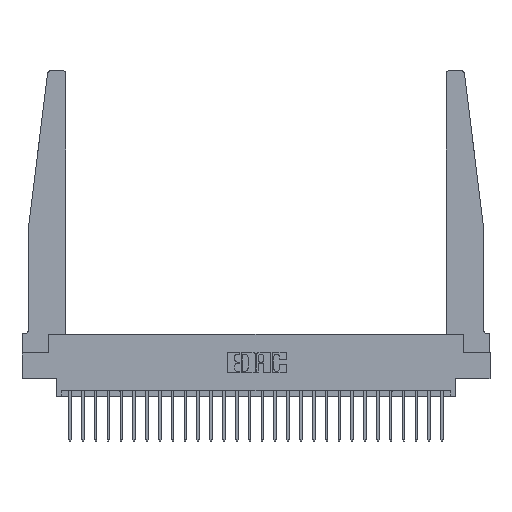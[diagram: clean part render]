
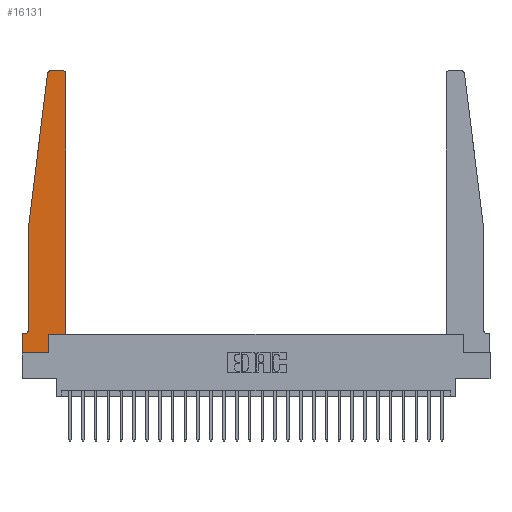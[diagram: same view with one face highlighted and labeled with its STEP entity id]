
A CAD part, top view. The second image highlights one B-rep face of the part: STEP entity #16131.
In plain terms, the highlighted planar face has unit normal (0, 0, 1).
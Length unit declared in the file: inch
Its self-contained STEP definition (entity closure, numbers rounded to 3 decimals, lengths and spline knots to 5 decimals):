
#276 = VECTOR ( 'NONE', #16497, 39.37008 ) ;
#402 = EDGE_CURVE ( 'NONE', #14051, #10019, #10716, .T. ) ;
#574 = ORIENTED_EDGE ( 'NONE', *, *, #2592, .T. ) ;
#743 = LINE ( 'NONE', #22726, #1393 ) ;
#865 = LINE ( 'NONE', #4766, #21819 ) ;
#1152 = CARTESIAN_POINT ( 'NONE',  ( 0.395, 2.75, 0.37 ) ) ;
#1393 = VECTOR ( 'NONE', #10576, 39.37008 ) ;
#1911 = EDGE_CURVE ( 'NONE', #15231, #13709, #19567, .T. ) ;
#2016 = AXIS2_PLACEMENT_3D ( 'NONE', #4565, #18829, #6612 ) ;
#2082 = VECTOR ( 'NONE', #21500, 39.37008 ) ;
#2258 = CARTESIAN_POINT ( 'NONE',  ( 0., 0., 0.37 ) ) ;
#2498 = ORIENTED_EDGE ( 'NONE', *, *, #7749, .T. ) ;
#2572 = CARTESIAN_POINT ( 'NONE',  ( 0., 0., 0.37 ) ) ;
#2592 = EDGE_CURVE ( 'NONE', #13709, #11650, #3611, .T. ) ;
#3297 = FACE_OUTER_BOUND ( 'NONE', #6999, .T. ) ;
#3611 = LINE ( 'NONE', #21758, #14441 ) ;
#3746 = ORIENTED_EDGE ( 'NONE', *, *, #12620, .T. ) ;
#4225 = CARTESIAN_POINT ( 'NONE',  ( 0., 0.1875, 0.37 ) ) ;
#4300 = VERTEX_POINT ( 'NONE', #16237 ) ;
#4429 = VECTOR ( 'NONE', #10445, 39.37008 ) ;
#4565 = CARTESIAN_POINT ( 'NONE',  ( 0.27653, 2.72, 0.37 ) ) ;
#4584 = DIRECTION ( 'NONE',  ( 0., -1., 0. ) ) ;
#4766 = CARTESIAN_POINT ( 'NONE',  ( 0.425, 0.18, 0.37 ) ) ;
#5009 = CARTESIAN_POINT ( 'NONE',  ( 0.015, 0.2375, 0.37 ) ) ;
#5012 = ORIENTED_EDGE ( 'NONE', *, *, #13566, .T. ) ;
#5018 = LINE ( 'NONE', #2258, #276 ) ;
#5101 = LINE ( 'NONE', #6433, #17252 ) ;
#5289 = AXIS2_PLACEMENT_3D ( 'NONE', #19246, #7040, #21251 ) ;
#5971 = ORIENTED_EDGE ( 'NONE', *, *, #9443, .T. ) ;
#6433 = CARTESIAN_POINT ( 'NONE',  ( 0.065, 1.25, 0.37 ) ) ;
#6599 = ORIENTED_EDGE ( 'NONE', *, *, #21748, .T. ) ;
#6612 = DIRECTION ( 'NONE',  ( 1., 0., 0. ) ) ;
#6999 = EDGE_LOOP ( 'NONE', ( #574, #5971, #6599, #12017, #22783, #2498, #13295, #3746, #9151, #19959, #5012, #15879 ) ) ;
#7040 = DIRECTION ( 'NONE',  ( 0., 0., 1. ) ) ;
#7749 = EDGE_CURVE ( 'NONE', #10019, #13974, #743, .T. ) ;
#7973 = CARTESIAN_POINT ( 'NONE',  ( 0., 0.1875, 0.37 ) ) ;
#8414 = CARTESIAN_POINT ( 'NONE',  ( 0.065, 1.25, 0.37 ) ) ;
#8613 = VERTEX_POINT ( 'NONE', #17256 ) ;
#8951 = EDGE_CURVE ( 'NONE', #20756, #14051, #5101, .T. ) ;
#9151 = ORIENTED_EDGE ( 'NONE', *, *, #14937, .T. ) ;
#9443 = EDGE_CURVE ( 'NONE', #11650, #11386, #11553, .T. ) ;
#9492 = VECTOR ( 'NONE', #4584, 39.37008 ) ;
#9989 = DIRECTION ( 'NONE',  ( 1., 0., 0. ) ) ;
#10019 = VERTEX_POINT ( 'NONE', #24514 ) ;
#10174 = CARTESIAN_POINT ( 'NONE',  ( 0.24675, 2.72367, 0.37 ) ) ;
#10445 = DIRECTION ( 'NONE',  ( -0.122, -0.992, 0. ) ) ;
#10576 = DIRECTION ( 'NONE',  ( -1., 0., 0. ) ) ;
#10716 = CIRCLE ( 'NONE', #11407, 0.05 ) ;
#11386 = VERTEX_POINT ( 'NONE', #10174 ) ;
#11407 = AXIS2_PLACEMENT_3D ( 'NONE', #5009, #18668, #23817 ) ;
#11553 = CIRCLE ( 'NONE', #2016, 0.03 ) ;
#11650 = VERTEX_POINT ( 'NONE', #21070 ) ;
#11752 = CARTESIAN_POINT ( 'NONE',  ( 0.065, 1.25, 0.37 ) ) ;
#11955 = PLANE ( 'NONE',  #14681 ) ;
#12017 = ORIENTED_EDGE ( 'NONE', *, *, #8951, .T. ) ;
#12620 = EDGE_CURVE ( 'NONE', #4300, #22200, #5018, .T. ) ;
#13295 = ORIENTED_EDGE ( 'NONE', *, *, #24982, .T. ) ;
#13436 = CARTESIAN_POINT ( 'NONE',  ( 0.2605, 0.18, 0.37 ) ) ;
#13566 = EDGE_CURVE ( 'NONE', #8613, #15231, #865, .T. ) ;
#13709 = VERTEX_POINT ( 'NONE', #1152 ) ;
#13938 = LINE ( 'NONE', #18996, #24018 ) ;
#13974 = VERTEX_POINT ( 'NONE', #4225 ) ;
#14051 = VERTEX_POINT ( 'NONE', #18653 ) ;
#14441 = VECTOR ( 'NONE', #23835, 39.37008 ) ;
#14681 = AXIS2_PLACEMENT_3D ( 'NONE', #7973, #22161, #9989 ) ;
#14937 = EDGE_CURVE ( 'NONE', #22200, #22851, #23606, .T. ) ;
#15231 = VERTEX_POINT ( 'NONE', #16384 ) ;
#15879 = ORIENTED_EDGE ( 'NONE', *, *, #1911, .T. ) ;
#15903 = CARTESIAN_POINT ( 'NONE',  ( 0.2605, 0., 0.37 ) ) ;
#16131 = ADVANCED_FACE ( 'NONE', ( #3297 ), #11955, .T. ) ;
#16237 = CARTESIAN_POINT ( 'NONE',  ( 0., 0., 0.37 ) ) ;
#16384 = CARTESIAN_POINT ( 'NONE',  ( 0.425, 2.72, 0.37 ) ) ;
#16497 = DIRECTION ( 'NONE',  ( 1., 0., 0. ) ) ;
#17252 = VECTOR ( 'NONE', #22672, 39.37008 ) ;
#17256 = CARTESIAN_POINT ( 'NONE',  ( 0.425, 0.18, 0.37 ) ) ;
#18190 = CARTESIAN_POINT ( 'NONE',  ( 0.2605, 0.18, 0.37 ) ) ;
#18653 = CARTESIAN_POINT ( 'NONE',  ( 0.065, 0.2375, 0.37 ) ) ;
#18668 = DIRECTION ( 'NONE',  ( 0., 0., -1. ) ) ;
#18829 = DIRECTION ( 'NONE',  ( 0., 0., 1. ) ) ;
#18996 = CARTESIAN_POINT ( 'NONE',  ( 0.425, 0.18, 0.37 ) ) ;
#19033 = DIRECTION ( 'NONE',  ( 0., 1., 0. ) ) ;
#19082 = DIRECTION ( 'NONE',  ( 1., 0., 0. ) ) ;
#19246 = CARTESIAN_POINT ( 'NONE',  ( 0.395, 2.72, 0.37 ) ) ;
#19401 = LINE ( 'NONE', #8414, #4429 ) ;
#19567 = CIRCLE ( 'NONE', #5289, 0.03 ) ;
#19959 = ORIENTED_EDGE ( 'NONE', *, *, #25769, .T. ) ;
#20756 = VERTEX_POINT ( 'NONE', #11752 ) ;
#21070 = CARTESIAN_POINT ( 'NONE',  ( 0.27653, 2.75, 0.37 ) ) ;
#21251 = DIRECTION ( 'NONE',  ( 1., 0., 0. ) ) ;
#21500 = DIRECTION ( 'NONE',  ( 0., 1., 0. ) ) ;
#21748 = EDGE_CURVE ( 'NONE', #11386, #20756, #19401, .T. ) ;
#21758 = CARTESIAN_POINT ( 'NONE',  ( 0.25, 2.75, 0.37 ) ) ;
#21819 = VECTOR ( 'NONE', #19033, 39.37008 ) ;
#22161 = DIRECTION ( 'NONE',  ( 0., 0., 1. ) ) ;
#22200 = VERTEX_POINT ( 'NONE', #15903 ) ;
#22672 = DIRECTION ( 'NONE',  ( 0., -1., 0. ) ) ;
#22726 = CARTESIAN_POINT ( 'NONE',  ( 0.065, 0.1875, 0.37 ) ) ;
#22783 = ORIENTED_EDGE ( 'NONE', *, *, #402, .T. ) ;
#22851 = VERTEX_POINT ( 'NONE', #18190 ) ;
#23606 = LINE ( 'NONE', #13436, #2082 ) ;
#23817 = DIRECTION ( 'NONE',  ( -1., 0., 0. ) ) ;
#23835 = DIRECTION ( 'NONE',  ( -1., 0., 0. ) ) ;
#24018 = VECTOR ( 'NONE', #19082, 39.37008 ) ;
#24514 = CARTESIAN_POINT ( 'NONE',  ( 0.015, 0.1875, 0.37 ) ) ;
#24982 = EDGE_CURVE ( 'NONE', #13974, #4300, #25565, .T. ) ;
#25565 = LINE ( 'NONE', #2572, #9492 ) ;
#25769 = EDGE_CURVE ( 'NONE', #22851, #8613, #13938, .T. ) ;
